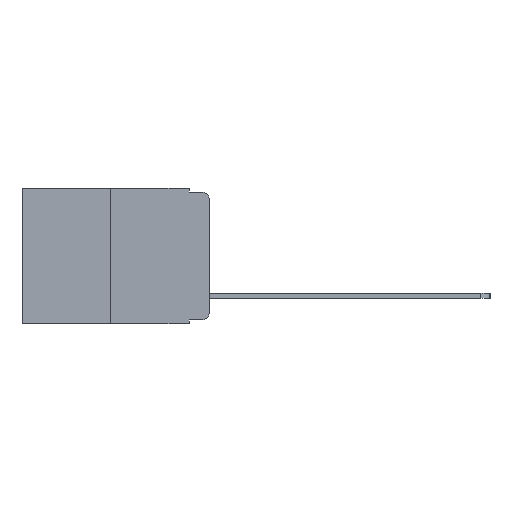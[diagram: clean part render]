
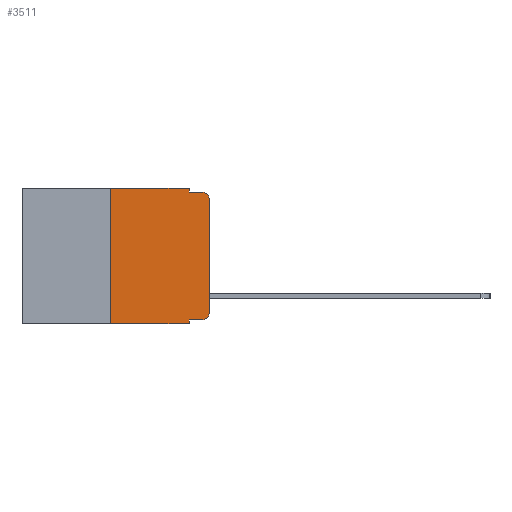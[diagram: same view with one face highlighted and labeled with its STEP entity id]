
A CAD part, left-side view. The second image highlights one B-rep face of the part: STEP entity #3511.
In plain terms, the highlighted planar face has unit normal (-1, 0, 0).
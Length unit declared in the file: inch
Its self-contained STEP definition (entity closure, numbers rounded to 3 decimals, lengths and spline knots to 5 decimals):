
#714 = LINE ( 'NONE', #17993, #21475 ) ;
#1344 = CARTESIAN_POINT ( 'NONE',  ( 0., 0.02, -0.313 ) ) ;
#1492 = CARTESIAN_POINT ( 'NONE',  ( 0., 0.051, -0.01 ) ) ;
#1780 = ORIENTED_EDGE ( 'NONE', *, *, #9729, .F. ) ;
#2263 = CARTESIAN_POINT ( 'NONE',  ( 0., 0.02, -0.333 ) ) ;
#2342 = EDGE_CURVE ( 'NONE', #24933, #6832, #20703, .T. ) ;
#2459 = LINE ( 'NONE', #9941, #17906 ) ;
#2812 = VERTEX_POINT ( 'NONE', #10021 ) ;
#3410 = VECTOR ( 'NONE', #23017, 39.37008 ) ;
#3451 = DIRECTION ( 'NONE',  ( 0., 0., -1. ) ) ;
#3511 = ADVANCED_FACE ( 'NONE', ( #8886 ), #21983, .F. ) ;
#3730 = EDGE_CURVE ( 'NONE', #20366, #6832, #4385, .T. ) ;
#4385 = CIRCLE ( 'NONE', #21593, 0.02 ) ;
#4710 = CARTESIAN_POINT ( 'NONE',  ( 0., 0.02, -0.01 ) ) ;
#6009 = ORIENTED_EDGE ( 'NONE', *, *, #22515, .F. ) ;
#6832 = VERTEX_POINT ( 'NONE', #4710 ) ;
#7036 = CARTESIAN_POINT ( 'NONE',  ( 0., 0.25, -0.343 ) ) ;
#7122 = DIRECTION ( 'NONE',  ( -1., 0., 0. ) ) ;
#7894 = VECTOR ( 'NONE', #17738, 39.37008 ) ;
#7978 = CARTESIAN_POINT ( 'NONE',  ( 0., 0.051, 0. ) ) ;
#8125 = CARTESIAN_POINT ( 'NONE',  ( 0., 0.25, 0. ) ) ;
#8886 = FACE_OUTER_BOUND ( 'NONE', #25178, .T. ) ;
#8906 = LINE ( 'NONE', #7978, #22810 ) ;
#9583 = LINE ( 'NONE', #13671, #14299 ) ;
#9602 = VERTEX_POINT ( 'NONE', #9733 ) ;
#9681 = AXIS2_PLACEMENT_3D ( 'NONE', #25779, #25865, #14196 ) ;
#9729 = EDGE_CURVE ( 'NONE', #11871, #20452, #24701, .T. ) ;
#9733 = CARTESIAN_POINT ( 'NONE',  ( 0., 0.051, 0. ) ) ;
#9849 = CARTESIAN_POINT ( 'NONE',  ( 0., 0.051, 0. ) ) ;
#9941 = CARTESIAN_POINT ( 'NONE',  ( 0., 0., 0. ) ) ;
#10021 = CARTESIAN_POINT ( 'NONE',  ( 0., 0., -0.313 ) ) ;
#10192 = DIRECTION ( 'NONE',  ( 0., 0., 1. ) ) ;
#10213 = EDGE_CURVE ( 'NONE', #11871, #14895, #9583, .T. ) ;
#10968 = EDGE_CURVE ( 'NONE', #2812, #20366, #2459, .T. ) ;
#11296 = CARTESIAN_POINT ( 'NONE',  ( 0., 0.051, -0.343 ) ) ;
#11871 = VERTEX_POINT ( 'NONE', #7036 ) ;
#12136 = CARTESIAN_POINT ( 'NONE',  ( 0., 0.051, -0.333 ) ) ;
#12644 = CARTESIAN_POINT ( 'NONE',  ( 0., 0.25, 0. ) ) ;
#12992 = ORIENTED_EDGE ( 'NONE', *, *, #3730, .T. ) ;
#13190 = CARTESIAN_POINT ( 'NONE',  ( 0., 0.473, 0. ) ) ;
#13247 = EDGE_CURVE ( 'NONE', #19912, #2812, #25583, .T. ) ;
#13671 = CARTESIAN_POINT ( 'NONE',  ( 0., 0.473, -0.343 ) ) ;
#14196 = DIRECTION ( 'NONE',  ( 0., 0., -1. ) ) ;
#14217 = LINE ( 'NONE', #13190, #3410 ) ;
#14299 = VECTOR ( 'NONE', #15564, 39.37008 ) ;
#14322 = VECTOR ( 'NONE', #10192, 39.37008 ) ;
#14895 = VERTEX_POINT ( 'NONE', #11296 ) ;
#15092 = EDGE_CURVE ( 'NONE', #9602, #24933, #23691, .T. ) ;
#15453 = ORIENTED_EDGE ( 'NONE', *, *, #2342, .F. ) ;
#15564 = DIRECTION ( 'NONE',  ( 0., -1., 0. ) ) ;
#15568 = DIRECTION ( 'NONE',  ( -1., 0., 0. ) ) ;
#15939 = DIRECTION ( 'NONE',  ( 0., 0., 1. ) ) ;
#17674 = DIRECTION ( 'NONE',  ( 0., -1., 0. ) ) ;
#17738 = DIRECTION ( 'NONE',  ( 0., 0., -1. ) ) ;
#17906 = VECTOR ( 'NONE', #15939, 39.37008 ) ;
#17993 = CARTESIAN_POINT ( 'NONE',  ( 0., 0.051, -0.333 ) ) ;
#18213 = CARTESIAN_POINT ( 'NONE',  ( 0., 0., -0.03 ) ) ;
#19083 = CARTESIAN_POINT ( 'NONE',  ( 0., 0.02, -0.03 ) ) ;
#19749 = ORIENTED_EDGE ( 'NONE', *, *, #22148, .F. ) ;
#19912 = VERTEX_POINT ( 'NONE', #2263 ) ;
#19961 = DIRECTION ( 'NONE',  ( 0., -1., 0. ) ) ;
#20077 = VECTOR ( 'NONE', #17674, 39.37008 ) ;
#20366 = VERTEX_POINT ( 'NONE', #18213 ) ;
#20452 = VERTEX_POINT ( 'NONE', #12644 ) ;
#20666 = ORIENTED_EDGE ( 'NONE', *, *, #15092, .F. ) ;
#20703 = LINE ( 'NONE', #1492, #20077 ) ;
#20981 = ORIENTED_EDGE ( 'NONE', *, *, #13247, .T. ) ;
#21046 = DIRECTION ( 'NONE',  ( 0., 0., -1. ) ) ;
#21475 = VECTOR ( 'NONE', #19961, 39.37008 ) ;
#21593 = AXIS2_PLACEMENT_3D ( 'NONE', #19083, #7122, #21046 ) ;
#21983 = PLANE ( 'NONE',  #9681 ) ;
#22148 = EDGE_CURVE ( 'NONE', #24558, #14895, #8906, .T. ) ;
#22515 = EDGE_CURVE ( 'NONE', #20452, #9602, #14217, .T. ) ;
#22781 = ORIENTED_EDGE ( 'NONE', *, *, #10968, .T. ) ;
#22810 = VECTOR ( 'NONE', #23808, 39.37008 ) ;
#23017 = DIRECTION ( 'NONE',  ( 0., -1., 0. ) ) ;
#23086 = ORIENTED_EDGE ( 'NONE', *, *, #10213, .T. ) ;
#23144 = CARTESIAN_POINT ( 'NONE',  ( 0., 0.051, -0.01 ) ) ;
#23691 = LINE ( 'NONE', #9849, #7894 ) ;
#23808 = DIRECTION ( 'NONE',  ( 0., 0., -1. ) ) ;
#23925 = EDGE_CURVE ( 'NONE', #24558, #19912, #714, .T. ) ;
#24558 = VERTEX_POINT ( 'NONE', #12136 ) ;
#24701 = LINE ( 'NONE', #8125, #14322 ) ;
#24899 = ORIENTED_EDGE ( 'NONE', *, *, #23925, .T. ) ;
#24933 = VERTEX_POINT ( 'NONE', #23144 ) ;
#25178 = EDGE_LOOP ( 'NONE', ( #22781, #12992, #15453, #20666, #6009, #1780, #23086, #19749, #24899, #20981 ) ) ;
#25273 = AXIS2_PLACEMENT_3D ( 'NONE', #1344, #15568, #3451 ) ;
#25583 = CIRCLE ( 'NONE', #25273, 0.02 ) ;
#25779 = CARTESIAN_POINT ( 'NONE',  ( 0., 0.473, 0. ) ) ;
#25865 = DIRECTION ( 'NONE',  ( 1., 0., 0. ) ) ;
